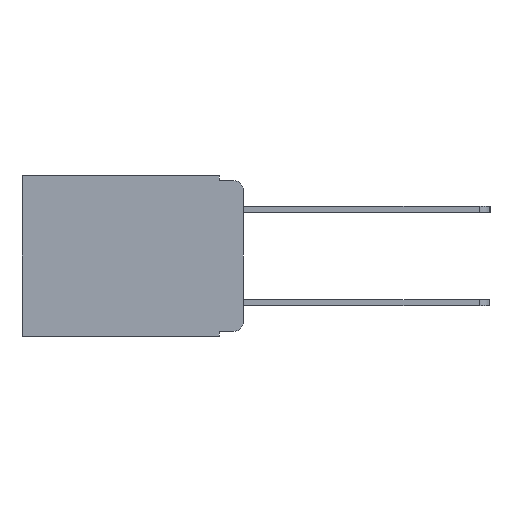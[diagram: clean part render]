
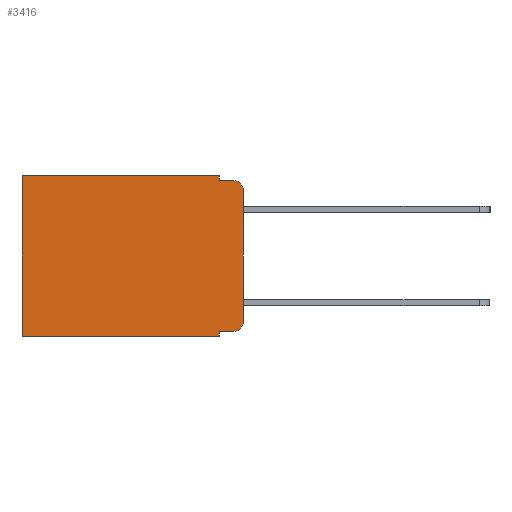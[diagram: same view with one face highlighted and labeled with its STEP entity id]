
A CAD part, left-side view. The second image highlights one B-rep face of the part: STEP entity #3416.
In plain terms, the highlighted planar face has unit normal (-1, 0, 0).
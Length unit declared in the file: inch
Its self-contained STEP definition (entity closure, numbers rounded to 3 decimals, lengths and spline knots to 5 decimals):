
#451 = CARTESIAN_POINT ( 'NONE',  ( 0.298, 0.473, -0.343 ) ) ;
#753 = CIRCLE ( 'NONE', #15229, 0.02 ) ;
#905 = ORIENTED_EDGE ( 'NONE', *, *, #8497, .F. ) ;
#1173 = ORIENTED_EDGE ( 'NONE', *, *, #10691, .T. ) ;
#1222 = CARTESIAN_POINT ( 'NONE',  ( 0.298, 0.02, -0.333 ) ) ;
#1309 = EDGE_LOOP ( 'NONE', ( #13204, #15070, #10227, #7444, #8976, #1173, #905, #11755, #9844, #16392 ) ) ;
#1338 = EDGE_CURVE ( 'NONE', #7519, #1620, #5951, .T. ) ;
#1620 = VERTEX_POINT ( 'NONE', #2694 ) ;
#2127 = LINE ( 'NONE', #2988, #5195 ) ;
#2144 = LINE ( 'NONE', #16936, #9440 ) ;
#2181 = DIRECTION ( 'NONE',  ( 0., 0., -1. ) ) ;
#2230 = VECTOR ( 'NONE', #18175, 39.37008 ) ;
#2249 = VERTEX_POINT ( 'NONE', #5529 ) ;
#2405 = VERTEX_POINT ( 'NONE', #1222 ) ;
#2694 = CARTESIAN_POINT ( 'NONE',  ( 0.298, 0., -0.313 ) ) ;
#2988 = CARTESIAN_POINT ( 'NONE',  ( 0.298, 0.051, -0.01 ) ) ;
#3416 = ADVANCED_FACE ( 'NONE', ( #17346 ), #5681, .F. ) ;
#3427 = VECTOR ( 'NONE', #2181, 39.37008 ) ;
#3491 = CARTESIAN_POINT ( 'NONE',  ( 0.298, 0., 0. ) ) ;
#3908 = CARTESIAN_POINT ( 'NONE',  ( 0.298, 0.02, -0.01 ) ) ;
#4399 = LINE ( 'NONE', #12177, #3427 ) ;
#4588 = DIRECTION ( 'NONE',  ( -1., 0., 0. ) ) ;
#4768 = VERTEX_POINT ( 'NONE', #4968 ) ;
#4925 = DIRECTION ( 'NONE',  ( 0., 1., 0. ) ) ;
#4968 = CARTESIAN_POINT ( 'NONE',  ( 0.298, 0.051, -0.333 ) ) ;
#5000 = DIRECTION ( 'NONE',  ( 0., 0., -1. ) ) ;
#5043 = DIRECTION ( 'NONE',  ( 0., 0., -1. ) ) ;
#5195 = VECTOR ( 'NONE', #11500, 39.37008 ) ;
#5383 = VERTEX_POINT ( 'NONE', #13664 ) ;
#5529 = CARTESIAN_POINT ( 'NONE',  ( 0.298, 0.051, -0.343 ) ) ;
#5540 = EDGE_CURVE ( 'NONE', #4768, #2405, #6213, .T. ) ;
#5681 = PLANE ( 'NONE',  #13732 ) ;
#5951 = LINE ( 'NONE', #3491, #15981 ) ;
#6087 = DIRECTION ( 'NONE',  ( 0., 1., 0. ) ) ;
#6213 = LINE ( 'NONE', #16785, #2230 ) ;
#6332 = CARTESIAN_POINT ( 'NONE',  ( 0.298, 0., 0. ) ) ;
#6438 = VERTEX_POINT ( 'NONE', #3908 ) ;
#6809 = AXIS2_PLACEMENT_3D ( 'NONE', #8422, #17822, #9811 ) ;
#6838 = LINE ( 'NONE', #9999, #13723 ) ;
#7444 = ORIENTED_EDGE ( 'NONE', *, *, #9797, .F. ) ;
#7493 = VECTOR ( 'NONE', #5043, 39.37008 ) ;
#7519 = VERTEX_POINT ( 'NONE', #14515 ) ;
#7800 = DIRECTION ( 'NONE',  ( 0., 0., -1. ) ) ;
#8085 = VERTEX_POINT ( 'NONE', #15761 ) ;
#8150 = VECTOR ( 'NONE', #4925, 39.37008 ) ;
#8156 = EDGE_CURVE ( 'NONE', #18226, #5383, #15348, .T. ) ;
#8422 = CARTESIAN_POINT ( 'NONE',  ( 0.298, 0.02, -0.313 ) ) ;
#8497 = EDGE_CURVE ( 'NONE', #2249, #15769, #2144, .T. ) ;
#8976 = ORIENTED_EDGE ( 'NONE', *, *, #8156, .T. ) ;
#9440 = VECTOR ( 'NONE', #6087, 39.37008 ) ;
#9797 = EDGE_CURVE ( 'NONE', #18226, #8085, #4399, .T. ) ;
#9811 = DIRECTION ( 'NONE',  ( 0., 0., -1. ) ) ;
#9844 = ORIENTED_EDGE ( 'NONE', *, *, #5540, .T. ) ;
#9999 = CARTESIAN_POINT ( 'NONE',  ( 0.298, 0.473, 0. ) ) ;
#10020 = DIRECTION ( 'NONE',  ( 1., 0., 0. ) ) ;
#10131 = EDGE_CURVE ( 'NONE', #7519, #6438, #753, .T. ) ;
#10227 = ORIENTED_EDGE ( 'NONE', *, *, #15539, .F. ) ;
#10691 = EDGE_CURVE ( 'NONE', #5383, #15769, #6838, .T. ) ;
#11370 = DIRECTION ( 'NONE',  ( 0., 0., -1. ) ) ;
#11500 = DIRECTION ( 'NONE',  ( 0., -1., 0. ) ) ;
#11755 = ORIENTED_EDGE ( 'NONE', *, *, #11941, .F. ) ;
#11941 = EDGE_CURVE ( 'NONE', #4768, #2249, #17830, .T. ) ;
#12177 = CARTESIAN_POINT ( 'NONE',  ( 0.298, 0.051, 0. ) ) ;
#12945 = CARTESIAN_POINT ( 'NONE',  ( 0.298, 0.02, -0.03 ) ) ;
#13204 = ORIENTED_EDGE ( 'NONE', *, *, #1338, .F. ) ;
#13664 = CARTESIAN_POINT ( 'NONE',  ( 0.298, 0.473, 0. ) ) ;
#13723 = VECTOR ( 'NONE', #11370, 39.37008 ) ;
#13732 = AXIS2_PLACEMENT_3D ( 'NONE', #18085, #10020, #7800 ) ;
#13880 = EDGE_CURVE ( 'NONE', #2405, #1620, #17959, .T. ) ;
#14283 = DIRECTION ( 'NONE',  ( 0., 0., -1. ) ) ;
#14515 = CARTESIAN_POINT ( 'NONE',  ( 0.298, 0., -0.03 ) ) ;
#14710 = CARTESIAN_POINT ( 'NONE',  ( 0.298, 0.051, 0. ) ) ;
#15070 = ORIENTED_EDGE ( 'NONE', *, *, #10131, .T. ) ;
#15229 = AXIS2_PLACEMENT_3D ( 'NONE', #12945, #4588, #14283 ) ;
#15348 = LINE ( 'NONE', #6332, #8150 ) ;
#15539 = EDGE_CURVE ( 'NONE', #8085, #6438, #2127, .T. ) ;
#15761 = CARTESIAN_POINT ( 'NONE',  ( 0.298, 0.051, -0.01 ) ) ;
#15769 = VERTEX_POINT ( 'NONE', #451 ) ;
#15981 = VECTOR ( 'NONE', #5000, 39.37008 ) ;
#16392 = ORIENTED_EDGE ( 'NONE', *, *, #13880, .T. ) ;
#16444 = CARTESIAN_POINT ( 'NONE',  ( 0.298, 0.051, 0. ) ) ;
#16785 = CARTESIAN_POINT ( 'NONE',  ( 0.298, 0.051, -0.333 ) ) ;
#16936 = CARTESIAN_POINT ( 'NONE',  ( 0.298, 0., -0.343 ) ) ;
#17346 = FACE_OUTER_BOUND ( 'NONE', #1309, .T. ) ;
#17822 = DIRECTION ( 'NONE',  ( -1., 0., 0. ) ) ;
#17830 = LINE ( 'NONE', #14710, #7493 ) ;
#17959 = CIRCLE ( 'NONE', #6809, 0.02 ) ;
#18085 = CARTESIAN_POINT ( 'NONE',  ( 0.298, 0., 0. ) ) ;
#18175 = DIRECTION ( 'NONE',  ( 0., -1., 0. ) ) ;
#18226 = VERTEX_POINT ( 'NONE', #16444 ) ;
